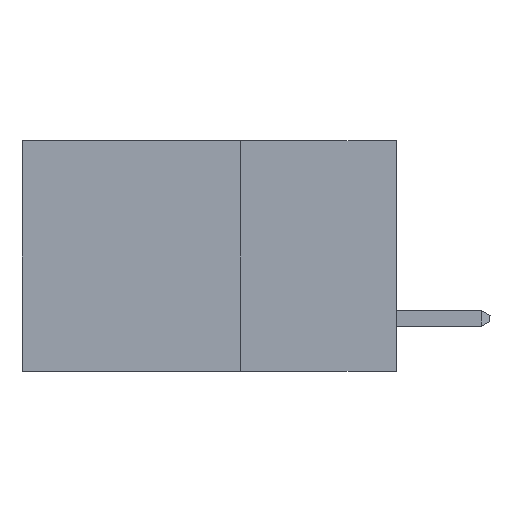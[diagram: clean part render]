
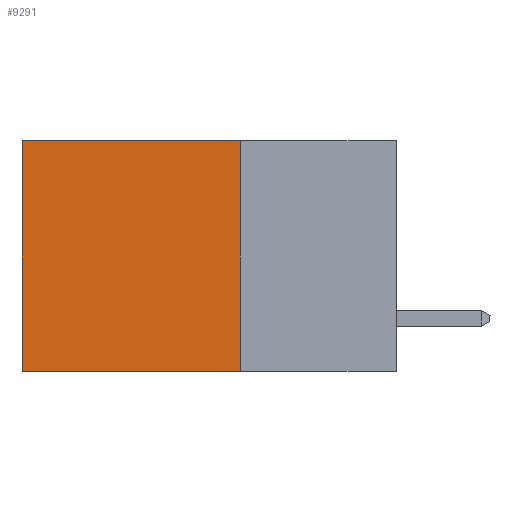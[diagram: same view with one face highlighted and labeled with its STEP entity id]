
A CAD part, left-side view. The second image highlights one B-rep face of the part: STEP entity #9291.
In plain terms, the highlighted planar face has unit normal (-1, 0, 0).
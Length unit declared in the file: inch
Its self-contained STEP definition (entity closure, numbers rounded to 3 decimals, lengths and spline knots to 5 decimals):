
#123 = EDGE_CURVE ( 'NONE', #7390, #4115, #5216, .T. ) ;
#350 = CARTESIAN_POINT ( 'NONE',  ( 0.2615, 0.6, 0. ) ) ;
#517 = CARTESIAN_POINT ( 'NONE',  ( 0.2615, 0.6, -0.37 ) ) ;
#1879 = EDGE_LOOP ( 'NONE', ( #7547, #6286, #11084, #8780 ) ) ;
#2579 = PLANE ( 'NONE',  #6084 ) ;
#2739 = DIRECTION ( 'NONE',  ( 0., 0., -1. ) ) ;
#3070 = LINE ( 'NONE', #517, #12047 ) ;
#3151 = EDGE_CURVE ( 'NONE', #7390, #15429, #12726, .T. ) ;
#3844 = DIRECTION ( 'NONE',  ( 0., 0., -1. ) ) ;
#3923 = VECTOR ( 'NONE', #10242, 39.37008 ) ;
#3927 = CARTESIAN_POINT ( 'NONE',  ( 0.2615, 0.25, -0.37 ) ) ;
#4115 = VERTEX_POINT ( 'NONE', #7051 ) ;
#4119 = CARTESIAN_POINT ( 'NONE',  ( 0.2615, 0.6, -0.37 ) ) ;
#5216 = LINE ( 'NONE', #3927, #7369 ) ;
#5233 = VERTEX_POINT ( 'NONE', #4119 ) ;
#5392 = DIRECTION ( 'NONE',  ( 0., 0., -1. ) ) ;
#6084 = AXIS2_PLACEMENT_3D ( 'NONE', #8588, #12102, #3844 ) ;
#6286 = ORIENTED_EDGE ( 'NONE', *, *, #6315, .F. ) ;
#6315 = EDGE_CURVE ( 'NONE', #4115, #5233, #12495, .T. ) ;
#7051 = CARTESIAN_POINT ( 'NONE',  ( 0.2615, 0.25, -0.37 ) ) ;
#7369 = VECTOR ( 'NONE', #2739, 39.37008 ) ;
#7390 = VERTEX_POINT ( 'NONE', #11401 ) ;
#7547 = ORIENTED_EDGE ( 'NONE', *, *, #15089, .T. ) ;
#8588 = CARTESIAN_POINT ( 'NONE',  ( 0.2615, 0.25, -0.37 ) ) ;
#8780 = ORIENTED_EDGE ( 'NONE', *, *, #3151, .T. ) ;
#9291 = ADVANCED_FACE ( 'NONE', ( #14819 ), #2579, .F. ) ;
#10242 = DIRECTION ( 'NONE',  ( 0., 1., 0. ) ) ;
#11084 = ORIENTED_EDGE ( 'NONE', *, *, #123, .F. ) ;
#11283 = CARTESIAN_POINT ( 'NONE',  ( 0.2615, 0.25, 0. ) ) ;
#11401 = CARTESIAN_POINT ( 'NONE',  ( 0.2615, 0.25, 0. ) ) ;
#12035 = DIRECTION ( 'NONE',  ( 0., 1., 0. ) ) ;
#12047 = VECTOR ( 'NONE', #5392, 39.37008 ) ;
#12102 = DIRECTION ( 'NONE',  ( 1., 0., 0. ) ) ;
#12119 = CARTESIAN_POINT ( 'NONE',  ( 0.2615, 0.25, -0.37 ) ) ;
#12495 = LINE ( 'NONE', #12119, #13718 ) ;
#12726 = LINE ( 'NONE', #11283, #3923 ) ;
#13718 = VECTOR ( 'NONE', #12035, 39.37008 ) ;
#14819 = FACE_OUTER_BOUND ( 'NONE', #1879, .T. ) ;
#15089 = EDGE_CURVE ( 'NONE', #15429, #5233, #3070, .T. ) ;
#15429 = VERTEX_POINT ( 'NONE', #350 ) ;
